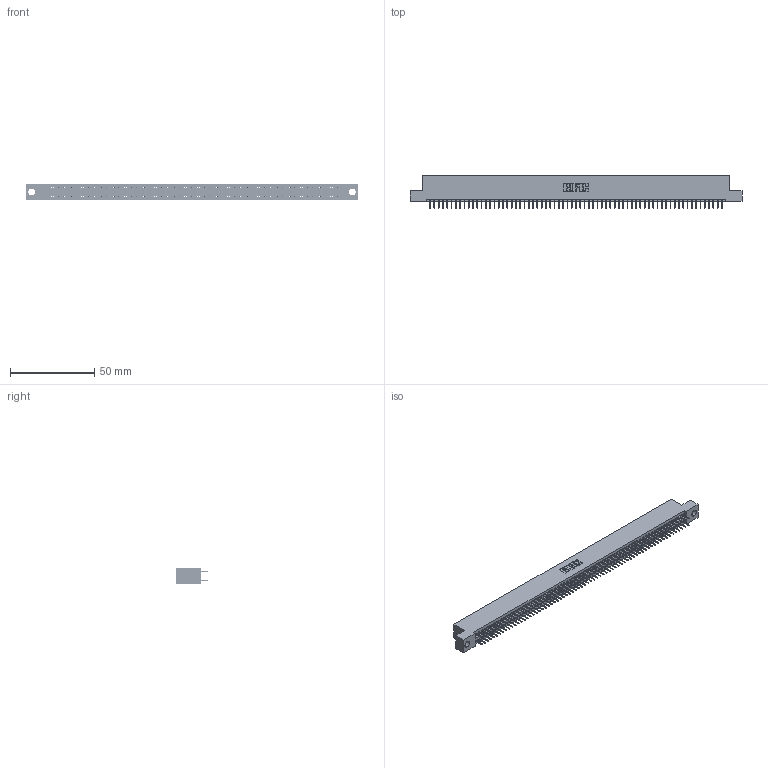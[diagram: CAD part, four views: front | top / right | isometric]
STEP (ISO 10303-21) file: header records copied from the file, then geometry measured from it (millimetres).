
FILE_DESCRIPTION (( 'STEP AP203' ), '1' );
FILE_NAME ('395-138-524-204.STEP', '2021-06-18T03:27:42', ( '' ), ( '' ), 'SwSTEP 2.0', 'SolidWorks 2020', '' );
FILE_SCHEMA (( 'CONFIG_CONTROL_DESIGN' ));
Length unit declared in the file: inch
Products named in the file (3): 345 Part_Flush Mounting Lugs - 0.156 Dia-TI; 345-292-001_345-293-124; 395-138-524-204
Assembly tree (139 placements, depth 2):
  395-138-524-204
    345 Part_Flush Mounting Lugs - 0.156 Dia-TI
    345-292-001_345-293-124  x138
Bounding box: 196.47 x 19.35 x 9.4 mm (x, y, z)
Volume: 19021 mm3; surface area: 27939.5 mm2
Topology: 139 solids, 139 shells, 7592 faces, 21491 edges, 13774 vertices
Faces by surface type: plane 5476, cylinder 2116
Entity records: 50997 total; most frequent: CARTESIAN_POINT 8526, ORIENTED_EDGE 8458, DIRECTION 7485, EDGE_CURVE 4229, LINE 3825, VECTOR 3825, VERTEX_POINT 2814, AXIS2_PLACEMENT_3D 1830
